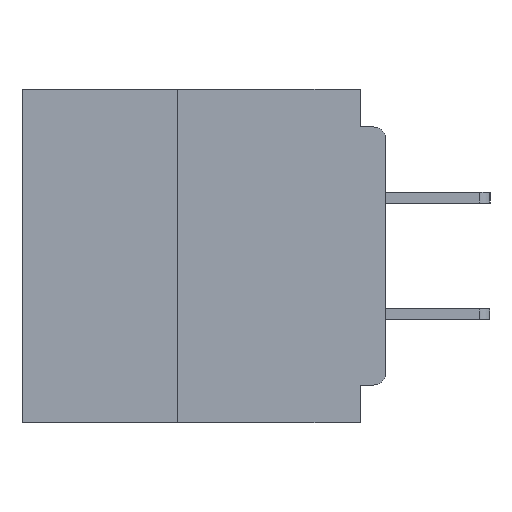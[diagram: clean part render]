
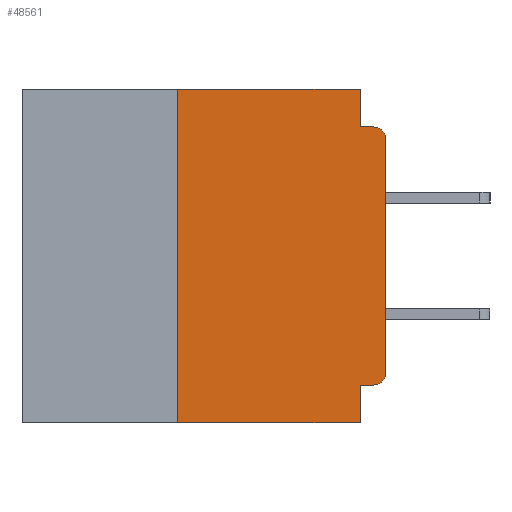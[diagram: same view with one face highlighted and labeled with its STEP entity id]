
A CAD part, left-side view. The second image highlights one B-rep face of the part: STEP entity #48561.
In plain terms, the highlighted planar face has unit normal (-1, 0, 0).
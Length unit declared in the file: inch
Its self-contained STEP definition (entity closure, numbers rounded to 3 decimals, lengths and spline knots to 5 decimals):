
#288 = EDGE_CURVE ( 'NONE', #16261, #32179, #737, .T. ) ;
#535 = ORIENTED_EDGE ( 'NONE', *, *, #37817, .T. ) ;
#737 = LINE ( 'NONE', #34980, #30898 ) ;
#830 = DIRECTION ( 'NONE',  ( 0., 0., -1. ) ) ;
#1445 = VERTEX_POINT ( 'NONE', #43447 ) ;
#1742 = CARTESIAN_POINT ( 'NONE',  ( 0., 0.015, -0.045 ) ) ;
#2689 = ORIENTED_EDGE ( 'NONE', *, *, #17846, .F. ) ;
#2768 = VERTEX_POINT ( 'NONE', #1742 ) ;
#3164 = VECTOR ( 'NONE', #15250, 39.37008 ) ;
#3206 = CARTESIAN_POINT ( 'NONE',  ( 0., 0., -0.045 ) ) ;
#3307 = VERTEX_POINT ( 'NONE', #28848 ) ;
#3484 = CARTESIAN_POINT ( 'NONE',  ( 0., 0., -0.06 ) ) ;
#5279 = CARTESIAN_POINT ( 'NONE',  ( 0., 0.031, -0.355 ) ) ;
#7059 = DIRECTION ( 'NONE',  ( 0., -1., 0. ) ) ;
#8632 = EDGE_CURVE ( 'NONE', #32179, #2768, #25950, .T. ) ;
#9040 = AXIS2_PLACEMENT_3D ( 'NONE', #33911, #15295, #41461 ) ;
#9259 = DIRECTION ( 'NONE',  ( 0., -1., 0. ) ) ;
#9851 = ORIENTED_EDGE ( 'NONE', *, *, #8632, .T. ) ;
#10377 = ORIENTED_EDGE ( 'NONE', *, *, #16521, .F. ) ;
#10706 = CARTESIAN_POINT ( 'NONE',  ( 0., 0.031, 0. ) ) ;
#10776 = LINE ( 'NONE', #16074, #19692 ) ;
#13242 = ORIENTED_EDGE ( 'NONE', *, *, #27393, .F. ) ;
#13819 = CARTESIAN_POINT ( 'NONE',  ( 0., 0.031, 0. ) ) ;
#15250 = DIRECTION ( 'NONE',  ( 0., 1., 0. ) ) ;
#15295 = DIRECTION ( 'NONE',  ( 1., 0., 0. ) ) ;
#15301 = LINE ( 'NONE', #13819, #35172 ) ;
#15513 = ORIENTED_EDGE ( 'NONE', *, *, #21796, .F. ) ;
#16028 = CARTESIAN_POINT ( 'NONE',  ( 0., 0.031, -0.4 ) ) ;
#16074 = CARTESIAN_POINT ( 'NONE',  ( 0., 0.437, 0. ) ) ;
#16121 = VECTOR ( 'NONE', #9259, 39.37008 ) ;
#16261 = VERTEX_POINT ( 'NONE', #18946 ) ;
#16521 = EDGE_CURVE ( 'NONE', #26614, #1445, #38505, .T. ) ;
#16592 = CARTESIAN_POINT ( 'NONE',  ( 0., 0.25, -0.4 ) ) ;
#16760 = DIRECTION ( 'NONE',  ( -1., 0., 0. ) ) ;
#17406 = VECTOR ( 'NONE', #27908, 39.37008 ) ;
#17846 = EDGE_CURVE ( 'NONE', #46766, #2768, #28408, .T. ) ;
#18938 = AXIS2_PLACEMENT_3D ( 'NONE', #39190, #16760, #42907 ) ;
#18946 = CARTESIAN_POINT ( 'NONE',  ( 0., 0., -0.34 ) ) ;
#19226 = FACE_OUTER_BOUND ( 'NONE', #20554, .T. ) ;
#19547 = DIRECTION ( 'NONE',  ( -1., 0., 0. ) ) ;
#19692 = VECTOR ( 'NONE', #20049, 39.37008 ) ;
#20049 = DIRECTION ( 'NONE',  ( 0., -1., 0. ) ) ;
#20416 = AXIS2_PLACEMENT_3D ( 'NONE', #41916, #19547, #45648 ) ;
#20554 = EDGE_LOOP ( 'NONE', ( #30382, #9851, #2689, #13242, #43757, #10377, #46257, #15513, #44846, #535 ) ) ;
#21705 = VECTOR ( 'NONE', #830, 39.37008 ) ;
#21796 = EDGE_CURVE ( 'NONE', #33015, #3307, #22878, .T. ) ;
#22878 = LINE ( 'NONE', #16028, #21705 ) ;
#23672 = CARTESIAN_POINT ( 'NONE',  ( 0., 0.015, -0.355 ) ) ;
#24224 = VERTEX_POINT ( 'NONE', #23672 ) ;
#25950 = CIRCLE ( 'NONE', #18938, 0.015 ) ;
#26444 = PLANE ( 'NONE',  #9040 ) ;
#26614 = VERTEX_POINT ( 'NONE', #34806 ) ;
#27245 = VECTOR ( 'NONE', #7059, 39.37008 ) ;
#27393 = EDGE_CURVE ( 'NONE', #43118, #46766, #15301, .T. ) ;
#27824 = EDGE_CURVE ( 'NONE', #1445, #43118, #10776, .T. ) ;
#27908 = DIRECTION ( 'NONE',  ( 0., 0., 1. ) ) ;
#27939 = EDGE_CURVE ( 'NONE', #26614, #3307, #44784, .T. ) ;
#28335 = CIRCLE ( 'NONE', #20416, 0.015 ) ;
#28408 = LINE ( 'NONE', #3206, #27245 ) ;
#28848 = CARTESIAN_POINT ( 'NONE',  ( 0., 0.031, -0.4 ) ) ;
#29951 = CARTESIAN_POINT ( 'NONE',  ( 0., 0., -0.355 ) ) ;
#30382 = ORIENTED_EDGE ( 'NONE', *, *, #288, .T. ) ;
#30898 = VECTOR ( 'NONE', #34944, 39.37008 ) ;
#30978 = CARTESIAN_POINT ( 'NONE',  ( 0., 0.031, -0.045 ) ) ;
#31742 = CARTESIAN_POINT ( 'NONE',  ( 0., 0.437, -0.4 ) ) ;
#32179 = VERTEX_POINT ( 'NONE', #3484 ) ;
#33015 = VERTEX_POINT ( 'NONE', #5279 ) ;
#33911 = CARTESIAN_POINT ( 'NONE',  ( 0., 0.437, 0. ) ) ;
#34806 = CARTESIAN_POINT ( 'NONE',  ( 0., 0.25, -0.4 ) ) ;
#34944 = DIRECTION ( 'NONE',  ( 0., 0., 1. ) ) ;
#34980 = CARTESIAN_POINT ( 'NONE',  ( 0., 0., 0. ) ) ;
#35172 = VECTOR ( 'NONE', #40023, 39.37008 ) ;
#35560 = LINE ( 'NONE', #29951, #3164 ) ;
#37817 = EDGE_CURVE ( 'NONE', #24224, #16261, #28335, .T. ) ;
#38505 = LINE ( 'NONE', #16592, #17406 ) ;
#39190 = CARTESIAN_POINT ( 'NONE',  ( 0., 0.015, -0.06 ) ) ;
#40023 = DIRECTION ( 'NONE',  ( 0., 0., -1. ) ) ;
#41461 = DIRECTION ( 'NONE',  ( 0., 0., -1. ) ) ;
#41916 = CARTESIAN_POINT ( 'NONE',  ( 0., 0.015, -0.34 ) ) ;
#42677 = EDGE_CURVE ( 'NONE', #24224, #33015, #35560, .T. ) ;
#42907 = DIRECTION ( 'NONE',  ( 0., 0., -1. ) ) ;
#43118 = VERTEX_POINT ( 'NONE', #10706 ) ;
#43447 = CARTESIAN_POINT ( 'NONE',  ( 0., 0.25, 0. ) ) ;
#43757 = ORIENTED_EDGE ( 'NONE', *, *, #27824, .F. ) ;
#44784 = LINE ( 'NONE', #31742, #16121 ) ;
#44846 = ORIENTED_EDGE ( 'NONE', *, *, #42677, .F. ) ;
#45648 = DIRECTION ( 'NONE',  ( 0., 0., -1. ) ) ;
#46257 = ORIENTED_EDGE ( 'NONE', *, *, #27939, .T. ) ;
#46766 = VERTEX_POINT ( 'NONE', #30978 ) ;
#48561 = ADVANCED_FACE ( 'NONE', ( #19226 ), #26444, .F. ) ;
